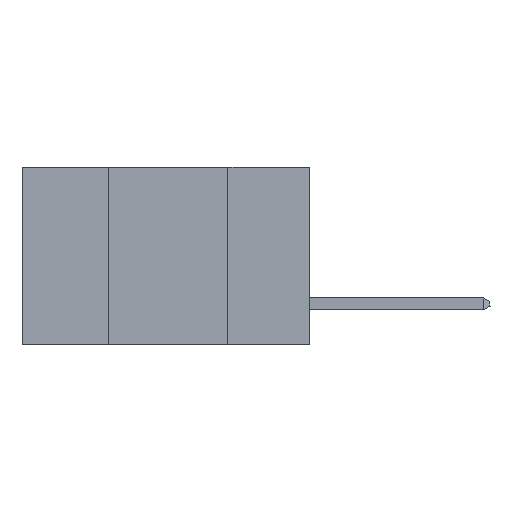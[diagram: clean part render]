
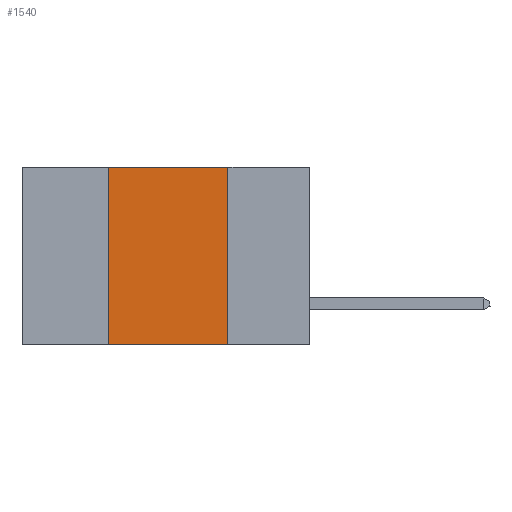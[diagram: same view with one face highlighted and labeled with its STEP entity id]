
A CAD part, left-side view. The second image highlights one B-rep face of the part: STEP entity #1540.
In plain terms, the highlighted planar face has unit normal (-1, 0, 0).
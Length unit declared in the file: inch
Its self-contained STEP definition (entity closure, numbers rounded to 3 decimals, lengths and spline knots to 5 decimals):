
#9 = LINE ( 'NONE', #17730, #6610 ) ;
#47 = VECTOR ( 'NONE', #6245, 39.37008 ) ;
#65 = VECTOR ( 'NONE', #17416, 39.37008 ) ;
#237 = DIRECTION ( 'NONE',  ( 0., -1., 0. ) ) ;
#436 = VERTEX_POINT ( 'NONE', #16552 ) ;
#934 = DIRECTION ( 'NONE',  ( 0., 0., 1. ) ) ;
#1540 = ADVANCED_FACE ( 'NONE', ( #9110 ), #8604, .F. ) ;
#1575 = EDGE_CURVE ( 'NONE', #16723, #16997, #15039, .T. ) ;
#3014 = CARTESIAN_POINT ( 'NONE',  ( 0., 0.6, -0.37 ) ) ;
#3536 = ORIENTED_EDGE ( 'NONE', *, *, #1575, .T. ) ;
#3775 = LINE ( 'NONE', #4775, #47 ) ;
#3883 = VECTOR ( 'NONE', #237, 39.37008 ) ;
#4440 = DIRECTION ( 'NONE',  ( 0., 0., -1. ) ) ;
#4775 = CARTESIAN_POINT ( 'NONE',  ( 0., 0.17, 0. ) ) ;
#4895 = CARTESIAN_POINT ( 'NONE',  ( 0., 0.6, 0. ) ) ;
#5216 = CARTESIAN_POINT ( 'NONE',  ( 0., 0.42, -0.37 ) ) ;
#5667 = ORIENTED_EDGE ( 'NONE', *, *, #17666, .F. ) ;
#6000 = LINE ( 'NONE', #4895, #65 ) ;
#6073 = ORIENTED_EDGE ( 'NONE', *, *, #8961, .F. ) ;
#6245 = DIRECTION ( 'NONE',  ( 0., 0., -1. ) ) ;
#6610 = VECTOR ( 'NONE', #934, 39.37008 ) ;
#8596 = EDGE_CURVE ( 'NONE', #436, #11087, #6000, .T. ) ;
#8604 = PLANE ( 'NONE',  #16223 ) ;
#8961 = EDGE_CURVE ( 'NONE', #11087, #16997, #3775, .T. ) ;
#9110 = FACE_OUTER_BOUND ( 'NONE', #14737, .T. ) ;
#10924 = CARTESIAN_POINT ( 'NONE',  ( 0., 0.17, 0. ) ) ;
#11087 = VERTEX_POINT ( 'NONE', #10924 ) ;
#12750 = CARTESIAN_POINT ( 'NONE',  ( 0., 0.6, 0. ) ) ;
#12803 = DIRECTION ( 'NONE',  ( 1., 0., 0. ) ) ;
#12911 = CARTESIAN_POINT ( 'NONE',  ( 0., 0.17, -0.37 ) ) ;
#13699 = ORIENTED_EDGE ( 'NONE', *, *, #8596, .F. ) ;
#14737 = EDGE_LOOP ( 'NONE', ( #6073, #13699, #5667, #3536 ) ) ;
#15039 = LINE ( 'NONE', #3014, #3883 ) ;
#16223 = AXIS2_PLACEMENT_3D ( 'NONE', #12750, #12803, #4440 ) ;
#16552 = CARTESIAN_POINT ( 'NONE',  ( 0., 0.42, 0. ) ) ;
#16723 = VERTEX_POINT ( 'NONE', #5216 ) ;
#16997 = VERTEX_POINT ( 'NONE', #12911 ) ;
#17416 = DIRECTION ( 'NONE',  ( 0., -1., 0. ) ) ;
#17666 = EDGE_CURVE ( 'NONE', #16723, #436, #9, .T. ) ;
#17730 = CARTESIAN_POINT ( 'NONE',  ( 0., 0.42, 0. ) ) ;
